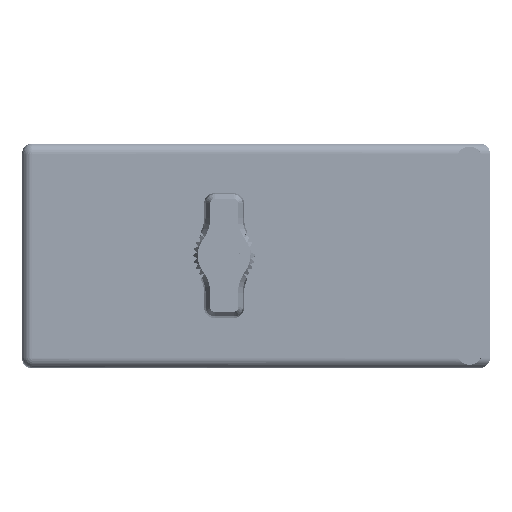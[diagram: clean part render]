
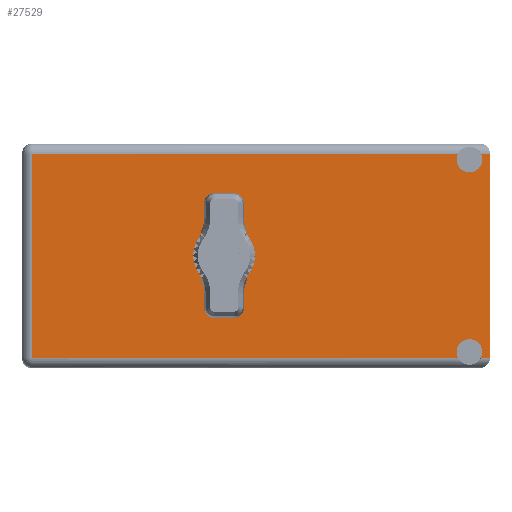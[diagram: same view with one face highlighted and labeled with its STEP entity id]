
A CAD part, top view. The second image highlights one B-rep face of the part: STEP entity #27529.
In plain terms, the highlighted face is planar.
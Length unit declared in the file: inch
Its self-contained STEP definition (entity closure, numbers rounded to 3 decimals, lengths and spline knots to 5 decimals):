
#121 = CIRCLE ( 'NONE', #29751, 0.0875 ) ;
#1227 = CARTESIAN_POINT ( 'NONE',  ( 1.6725, 1.93, 0.656 ) ) ;
#4832 = ORIENTED_EDGE ( 'NONE', *, *, #96215, .F. ) ;
#4927 = EDGE_CURVE ( 'NONE', #55578, #86990, #95825, .T. ) ;
#6457 = CARTESIAN_POINT ( 'NONE',  ( 1.75083, 1.93, 0.695 ) ) ;
#6851 = VERTEX_POINT ( 'NONE', #74084 ) ;
#7922 = DIRECTION ( 'NONE',  ( 0., 0., 1. ) ) ;
#9359 = CIRCLE ( 'NONE', #102342, 0.0875 ) ;
#9515 = CARTESIAN_POINT ( 'NONE',  ( 1.6725, 1.93, 0.5685 ) ) ;
#9711 = AXIS2_PLACEMENT_3D ( 'NONE', #78751, #33828, #114652 ) ;
#9759 = CARTESIAN_POINT ( 'NONE',  ( 1.8125, 1.93, 0.695 ) ) ;
#10279 = ORIENTED_EDGE ( 'NONE', *, *, #103251, .T. ) ;
#13172 = LINE ( 'NONE', #108563, #105466 ) ;
#13527 = CARTESIAN_POINT ( 'NONE',  ( 1.8125, 1.93, 0.695 ) ) ;
#13585 = EDGE_CURVE ( 'NONE', #74905, #48978, #97699, .T. ) ;
#14107 = VECTOR ( 'NONE', #76925, 39.37008 ) ;
#14848 = CARTESIAN_POINT ( 'NONE',  ( 1.6725, 1.93, -0.5685 ) ) ;
#15105 = DIRECTION ( 'NONE',  ( 0., 1., 0. ) ) ;
#15483 = ORIENTED_EDGE ( 'NONE', *, *, #16867, .F. ) ;
#16531 = DIRECTION ( 'NONE',  ( 0., 1., 0. ) ) ;
#16633 = CARTESIAN_POINT ( 'NONE',  ( 1.8125, 1.93, 0.765 ) ) ;
#16867 = EDGE_CURVE ( 'NONE', #43353, #53838, #22851, .T. ) ;
#19224 = DIRECTION ( 'NONE',  ( 0., 1., 0. ) ) ;
#21182 = ORIENTED_EDGE ( 'NONE', *, *, #56046, .T. ) ;
#22851 = CIRCLE ( 'NONE', #97160, 0.0875 ) ;
#25080 = AXIS2_PLACEMENT_3D ( 'NONE', #1227, #19224, #73490 ) ;
#26036 = CARTESIAN_POINT ( 'NONE',  ( 1.6725, 1.93, -0.656 ) ) ;
#27529 = ADVANCED_FACE ( 'NONE', ( #27997, #88089 ), #42123, .T. ) ;
#27989 = EDGE_CURVE ( 'NONE', #6851, #44906, #40405, .T. ) ;
#27997 = FACE_BOUND ( 'NONE', #49181, .T. ) ;
#28007 = ORIENTED_EDGE ( 'NONE', *, *, #63061, .T. ) ;
#29275 = DIRECTION ( 'NONE',  ( -1., 0., 0. ) ) ;
#29614 = ORIENTED_EDGE ( 'NONE', *, *, #96298, .F. ) ;
#29710 = AXIS2_PLACEMENT_3D ( 'NONE', #53246, #115706, #114575 ) ;
#29751 = AXIS2_PLACEMENT_3D ( 'NONE', #26036, #97508, #106471 ) ;
#33629 = LINE ( 'NONE', #94184, #14107 ) ;
#33659 = LINE ( 'NONE', #16633, #75571 ) ;
#33828 = DIRECTION ( 'NONE',  ( 0., 1., 0. ) ) ;
#34350 = CARTESIAN_POINT ( 'NONE',  ( -1.3775, 1.93, -0.765 ) ) ;
#38577 = CARTESIAN_POINT ( 'NONE',  ( 1.59417, 1.93, 0.695 ) ) ;
#39638 = LINE ( 'NONE', #9759, #99753 ) ;
#40286 = VECTOR ( 'NONE', #63209, 39.37008 ) ;
#40405 = CIRCLE ( 'NONE', #9711, 0.17 ) ;
#40736 = CARTESIAN_POINT ( 'NONE',  ( -1.3075, 1.93, 0.695 ) ) ;
#42123 = PLANE ( 'NONE',  #107780 ) ;
#43353 = VERTEX_POINT ( 'NONE', #44452 ) ;
#44452 = CARTESIAN_POINT ( 'NONE',  ( 1.59417, 1.93, -0.695 ) ) ;
#44906 = VERTEX_POINT ( 'NONE', #72211 ) ;
#46073 = EDGE_CURVE ( 'NONE', #98791, #55578, #9359, .T. ) ;
#46436 = DIRECTION ( 'NONE',  ( 1., 0., 0. ) ) ;
#48312 = ORIENTED_EDGE ( 'NONE', *, *, #27989, .F. ) ;
#48978 = VERTEX_POINT ( 'NONE', #60286 ) ;
#49181 = EDGE_LOOP ( 'NONE', ( #48312, #100574 ) ) ;
#50071 = ORIENTED_EDGE ( 'NONE', *, *, #13585, .T. ) ;
#50124 = VECTOR ( 'NONE', #57359, 39.37008 ) ;
#53006 = EDGE_CURVE ( 'NONE', #98791, #58669, #110148, .T. ) ;
#53246 = CARTESIAN_POINT ( 'NONE',  ( 0., 1.93, 0. ) ) ;
#53838 = VERTEX_POINT ( 'NONE', #14848 ) ;
#54225 = CARTESIAN_POINT ( 'NONE',  ( 1.8125, 1.93, 0.695 ) ) ;
#55578 = VERTEX_POINT ( 'NONE', #9515 ) ;
#56046 = EDGE_CURVE ( 'NONE', #80231, #86990, #39638, .T. ) ;
#56970 = CARTESIAN_POINT ( 'NONE',  ( -1.3775, 1.93, -0.695 ) ) ;
#57359 = DIRECTION ( 'NONE',  ( -1., 0., 0. ) ) ;
#58669 = VERTEX_POINT ( 'NONE', #13527 ) ;
#59447 = VERTEX_POINT ( 'NONE', #59616 ) ;
#59616 = CARTESIAN_POINT ( 'NONE',  ( -1.3075, 1.93, -0.695 ) ) ;
#59995 = ORIENTED_EDGE ( 'NONE', *, *, #53006, .T. ) ;
#60286 = CARTESIAN_POINT ( 'NONE',  ( 1.75083, 1.93, -0.695 ) ) ;
#63061 = EDGE_CURVE ( 'NONE', #43353, #59447, #13172, .T. ) ;
#63209 = DIRECTION ( 'NONE',  ( 1., 0., 0. ) ) ;
#70160 = ORIENTED_EDGE ( 'NONE', *, *, #46073, .F. ) ;
#70220 = DIRECTION ( 'NONE',  ( -1., 0., 0. ) ) ;
#72211 = CARTESIAN_POINT ( 'NONE',  ( 0., 1.93, -0.17 ) ) ;
#73490 = DIRECTION ( 'NONE',  ( 0., 0., 1. ) ) ;
#74084 = CARTESIAN_POINT ( 'NONE',  ( 0., 1.93, 0.17 ) ) ;
#74905 = VERTEX_POINT ( 'NONE', #80785 ) ;
#75571 = VECTOR ( 'NONE', #114660, 39.37008 ) ;
#76825 = CARTESIAN_POINT ( 'NONE',  ( 1.6725, 1.93, -0.656 ) ) ;
#76925 = DIRECTION ( 'NONE',  ( 0., 0., 1. ) ) ;
#78297 = CIRCLE ( 'NONE', #29710, 0.17 ) ;
#78751 = CARTESIAN_POINT ( 'NONE',  ( 0., 1.93, 0. ) ) ;
#80231 = VERTEX_POINT ( 'NONE', #40736 ) ;
#80785 = CARTESIAN_POINT ( 'NONE',  ( 1.8125, 1.93, -0.695 ) ) ;
#82024 = ORIENTED_EDGE ( 'NONE', *, *, #4927, .F. ) ;
#86866 = CARTESIAN_POINT ( 'NONE',  ( 1.6725, 1.93, 0.656 ) ) ;
#86990 = VERTEX_POINT ( 'NONE', #38577 ) ;
#88089 = FACE_OUTER_BOUND ( 'NONE', #105041, .T. ) ;
#88911 = EDGE_CURVE ( 'NONE', #44906, #6851, #78297, .T. ) ;
#94184 = CARTESIAN_POINT ( 'NONE',  ( -1.3075, 1.93, -0.765 ) ) ;
#95825 = CIRCLE ( 'NONE', #25080, 0.0875 ) ;
#96215 = EDGE_CURVE ( 'NONE', #74905, #58669, #33659, .T. ) ;
#96298 = EDGE_CURVE ( 'NONE', #53838, #48978, #121, .T. ) ;
#96868 = DIRECTION ( 'NONE',  ( 0., 1., 0. ) ) ;
#97160 = AXIS2_PLACEMENT_3D ( 'NONE', #76825, #15105, #104216 ) ;
#97508 = DIRECTION ( 'NONE',  ( 0., 1., 0. ) ) ;
#97699 = LINE ( 'NONE', #56970, #50124 ) ;
#98791 = VERTEX_POINT ( 'NONE', #6457 ) ;
#99753 = VECTOR ( 'NONE', #46436, 39.37008 ) ;
#100574 = ORIENTED_EDGE ( 'NONE', *, *, #88911, .F. ) ;
#102342 = AXIS2_PLACEMENT_3D ( 'NONE', #86866, #16531, #7922 ) ;
#103251 = EDGE_CURVE ( 'NONE', #59447, #80231, #33629, .T. ) ;
#104216 = DIRECTION ( 'NONE',  ( 0., 0., 1. ) ) ;
#105041 = EDGE_LOOP ( 'NONE', ( #21182, #82024, #70160, #59995, #4832, #50071, #29614, #15483, #28007, #10279 ) ) ;
#105466 = VECTOR ( 'NONE', #29275, 39.37008 ) ;
#106471 = DIRECTION ( 'NONE',  ( 0., 0., 1. ) ) ;
#107780 = AXIS2_PLACEMENT_3D ( 'NONE', #34350, #96868, #70220 ) ;
#108563 = CARTESIAN_POINT ( 'NONE',  ( -1.3775, 1.93, -0.695 ) ) ;
#110148 = LINE ( 'NONE', #54225, #40286 ) ;
#114575 = DIRECTION ( 'NONE',  ( 0., 0., 1. ) ) ;
#114652 = DIRECTION ( 'NONE',  ( 0., 0., 1. ) ) ;
#114660 = DIRECTION ( 'NONE',  ( 0., 0., 1. ) ) ;
#115706 = DIRECTION ( 'NONE',  ( 0., 1., 0. ) ) ;
